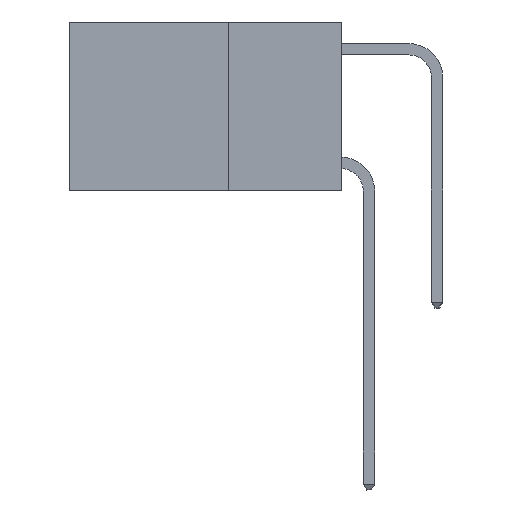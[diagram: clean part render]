
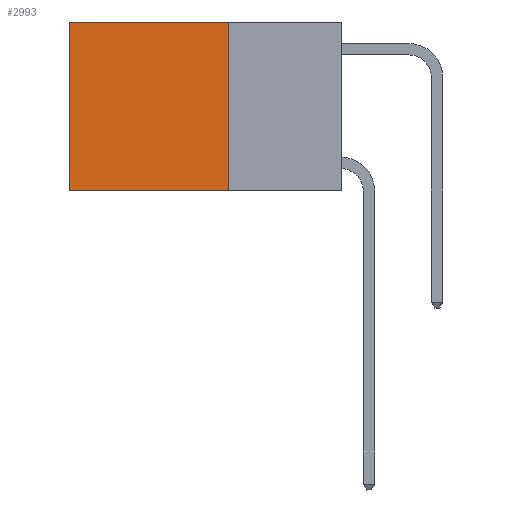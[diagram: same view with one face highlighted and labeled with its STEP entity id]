
A CAD part, left-side view. The second image highlights one B-rep face of the part: STEP entity #2993.
In plain terms, the highlighted planar face has unit normal (-1, 0, 0).
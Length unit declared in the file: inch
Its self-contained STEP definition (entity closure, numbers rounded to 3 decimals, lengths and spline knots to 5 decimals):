
#171 = ORIENTED_EDGE ( 'NONE', *, *, #13413, .T. ) ;
#210 = EDGE_LOOP ( 'NONE', ( #171, #3763, #10836, #8397 ) ) ;
#299 = LINE ( 'NONE', #7687, #13416 ) ;
#1380 = VECTOR ( 'NONE', #6399, 39.37008 ) ;
#1520 = VECTOR ( 'NONE', #14762, 39.37008 ) ;
#1647 = VECTOR ( 'NONE', #14545, 39.37008 ) ;
#2993 = ADVANCED_FACE ( 'NONE', ( #12404 ), #12965, .F. ) ;
#3763 = ORIENTED_EDGE ( 'NONE', *, *, #11832, .F. ) ;
#3903 = DIRECTION ( 'NONE',  ( 0., 1., 0. ) ) ;
#4783 = CARTESIAN_POINT ( 'NONE',  ( 0.2625, 0.6, 0. ) ) ;
#5161 = VERTEX_POINT ( 'NONE', #4783 ) ;
#5403 = CARTESIAN_POINT ( 'NONE',  ( 0.2625, 0.25, 0. ) ) ;
#5485 = CARTESIAN_POINT ( 'NONE',  ( 0.2625, 0.6, -0.37 ) ) ;
#6399 = DIRECTION ( 'NONE',  ( 0., 1., 0. ) ) ;
#6673 = DIRECTION ( 'NONE',  ( 1., 0., 0. ) ) ;
#7001 = CARTESIAN_POINT ( 'NONE',  ( 0.2625, 0.25, 0. ) ) ;
#7687 = CARTESIAN_POINT ( 'NONE',  ( 0.2625, 0.25, 0. ) ) ;
#8088 = EDGE_CURVE ( 'NONE', #14509, #15382, #8464, .T. ) ;
#8397 = ORIENTED_EDGE ( 'NONE', *, *, #14858, .T. ) ;
#8464 = LINE ( 'NONE', #7001, #1647 ) ;
#8484 = CARTESIAN_POINT ( 'NONE',  ( 0.2625, 0.6, 0. ) ) ;
#8605 = LINE ( 'NONE', #13951, #1380 ) ;
#9220 = AXIS2_PLACEMENT_3D ( 'NONE', #5403, #6673, #15481 ) ;
#9400 = CARTESIAN_POINT ( 'NONE',  ( 0.2625, 0.25, 0. ) ) ;
#10836 = ORIENTED_EDGE ( 'NONE', *, *, #8088, .F. ) ;
#11832 = EDGE_CURVE ( 'NONE', #15382, #15654, #8605, .T. ) ;
#12404 = FACE_OUTER_BOUND ( 'NONE', #210, .T. ) ;
#12521 = CARTESIAN_POINT ( 'NONE',  ( 0.2625, 0.25, -0.37 ) ) ;
#12965 = PLANE ( 'NONE',  #9220 ) ;
#13413 = EDGE_CURVE ( 'NONE', #5161, #15654, #15429, .T. ) ;
#13416 = VECTOR ( 'NONE', #3903, 39.37008 ) ;
#13951 = CARTESIAN_POINT ( 'NONE',  ( 0.2625, 0.25, -0.37 ) ) ;
#14509 = VERTEX_POINT ( 'NONE', #9400 ) ;
#14545 = DIRECTION ( 'NONE',  ( 0., 0., -1. ) ) ;
#14762 = DIRECTION ( 'NONE',  ( 0., 0., -1. ) ) ;
#14858 = EDGE_CURVE ( 'NONE', #14509, #5161, #299, .T. ) ;
#15382 = VERTEX_POINT ( 'NONE', #12521 ) ;
#15429 = LINE ( 'NONE', #8484, #1520 ) ;
#15481 = DIRECTION ( 'NONE',  ( 0., 0., -1. ) ) ;
#15654 = VERTEX_POINT ( 'NONE', #5485 ) ;
